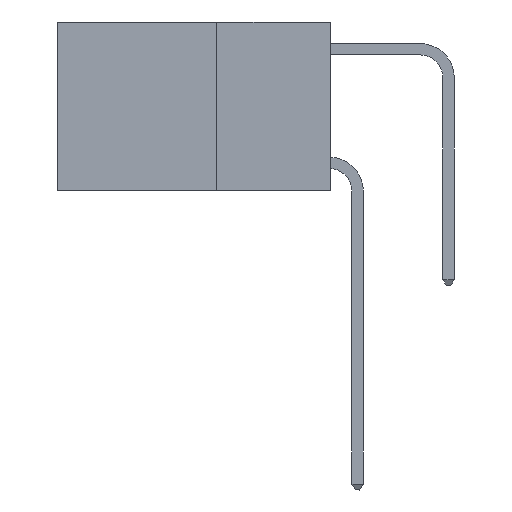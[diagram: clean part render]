
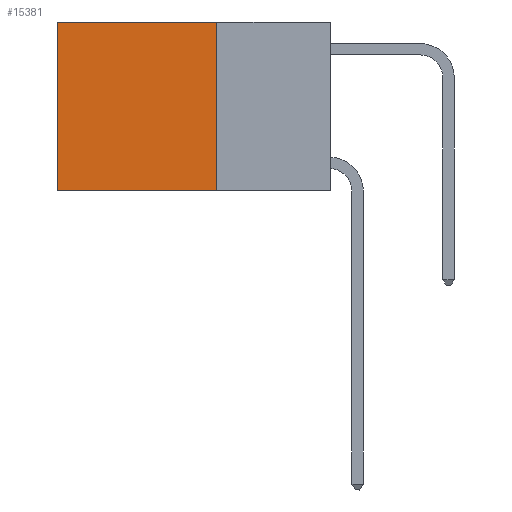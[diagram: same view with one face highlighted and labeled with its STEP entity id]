
A CAD part, left-side view. The second image highlights one B-rep face of the part: STEP entity #15381.
In plain terms, the highlighted planar face has unit normal (-1, 0, 0).
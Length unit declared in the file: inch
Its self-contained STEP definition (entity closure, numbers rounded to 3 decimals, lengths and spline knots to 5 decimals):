
#21 = VERTEX_POINT ( 'NONE', #3739 ) ;
#497 = AXIS2_PLACEMENT_3D ( 'NONE', #13332, #17983, #4081 ) ;
#760 = VERTEX_POINT ( 'NONE', #7599 ) ;
#1970 = VECTOR ( 'NONE', #8492, 39.37008 ) ;
#3284 = DIRECTION ( 'NONE',  ( 0., 0., -1. ) ) ;
#3447 = CARTESIAN_POINT ( 'NONE',  ( 0.2625, 0.25, 0. ) ) ;
#3460 = CARTESIAN_POINT ( 'NONE',  ( 0.2625, 0.25, 0. ) ) ;
#3537 = EDGE_LOOP ( 'NONE', ( #8966, #13050, #5348, #17692 ) ) ;
#3739 = CARTESIAN_POINT ( 'NONE',  ( 0.2625, 0.6, 0. ) ) ;
#4081 = DIRECTION ( 'NONE',  ( 0., 0., -1. ) ) ;
#4489 = LINE ( 'NONE', #14120, #15837 ) ;
#4514 = EDGE_CURVE ( 'NONE', #760, #17201, #14437, .T. ) ;
#5063 = DIRECTION ( 'NONE',  ( 0., 0., -1. ) ) ;
#5348 = ORIENTED_EDGE ( 'NONE', *, *, #11934, .F. ) ;
#6565 = FACE_OUTER_BOUND ( 'NONE', #3537, .T. ) ;
#6949 = CARTESIAN_POINT ( 'NONE',  ( 0.2625, 0.25, -0.37 ) ) ;
#6950 = VERTEX_POINT ( 'NONE', #15958 ) ;
#7599 = CARTESIAN_POINT ( 'NONE',  ( 0.2625, 0.25, -0.37 ) ) ;
#8357 = LINE ( 'NONE', #3460, #11952 ) ;
#8492 = DIRECTION ( 'NONE',  ( 0., 1., 0. ) ) ;
#8966 = ORIENTED_EDGE ( 'NONE', *, *, #17037, .T. ) ;
#9742 = LINE ( 'NONE', #3447, #17487 ) ;
#10115 = CARTESIAN_POINT ( 'NONE',  ( 0.2625, 0.6, -0.37 ) ) ;
#11812 = PLANE ( 'NONE',  #497 ) ;
#11934 = EDGE_CURVE ( 'NONE', #6950, #760, #9742, .T. ) ;
#11952 = VECTOR ( 'NONE', #12754, 39.37008 ) ;
#12754 = DIRECTION ( 'NONE',  ( 0., 1., 0. ) ) ;
#13050 = ORIENTED_EDGE ( 'NONE', *, *, #4514, .F. ) ;
#13332 = CARTESIAN_POINT ( 'NONE',  ( 0.2625, 0.25, 0. ) ) ;
#14120 = CARTESIAN_POINT ( 'NONE',  ( 0.2625, 0.6, 0. ) ) ;
#14437 = LINE ( 'NONE', #6949, #1970 ) ;
#15381 = ADVANCED_FACE ( 'NONE', ( #6565 ), #11812, .F. ) ;
#15837 = VECTOR ( 'NONE', #3284, 39.37008 ) ;
#15958 = CARTESIAN_POINT ( 'NONE',  ( 0.2625, 0.25, 0. ) ) ;
#17037 = EDGE_CURVE ( 'NONE', #21, #17201, #4489, .T. ) ;
#17201 = VERTEX_POINT ( 'NONE', #10115 ) ;
#17487 = VECTOR ( 'NONE', #5063, 39.37008 ) ;
#17692 = ORIENTED_EDGE ( 'NONE', *, *, #17899, .T. ) ;
#17899 = EDGE_CURVE ( 'NONE', #6950, #21, #8357, .T. ) ;
#17983 = DIRECTION ( 'NONE',  ( 1., 0., 0. ) ) ;
